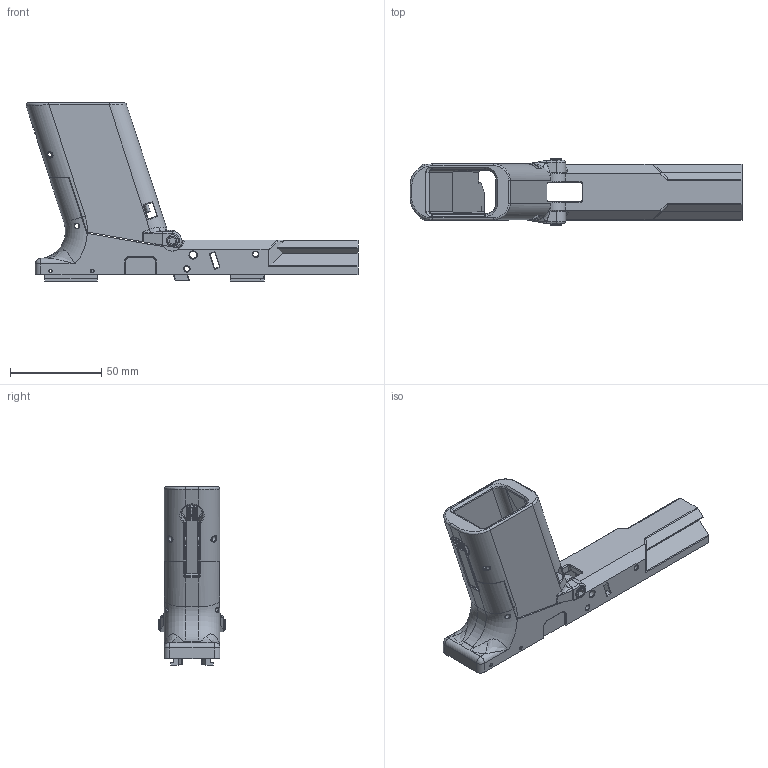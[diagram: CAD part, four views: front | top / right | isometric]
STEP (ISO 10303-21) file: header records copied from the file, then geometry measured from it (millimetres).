
FILE_DESCRIPTION(/* description */ (''),/* implementation_level */ '2;1');
FILE_NAME(/* name */ 'G19 FOLDING X FIXED.stp',/* time_stamp */ '2019-11-15T10:02:00+02:00',/* author */ (''),/* organization */ (''),/* preprocessor_version */ 'ST-DEVELOPER v15.2',/* originating_system */ 'Autodesk Translator Framework v2.0.0.5431',/* authorisation */ '');
FILE_SCHEMA (('AUTOMOTIVE_DESIGN { 1 0 10303 214 3 1 1 }'));
Length unit declared in the file: centimetre
Products named in the file (1): FOLDING X V5 FIXED
Bounding box: 181.62 x 36.6 x 97.38 mm (x, y, z)
Volume: 97898.8 mm3; surface area: 54978.3 mm2
Topology: 10 solids, 11 shells, 1273 faces, 3184 edges, 1898 vertices
Faces by surface type: cylinder 473, plane 355, bspline 222, torus 127, sphere 52, cone 44
Full cylindrical faces by diameter (mm): 1.655 x8, 1.8 x1, 2.557 x2, 3 x7, 3.057 x4, 3.06 x3, 4 x1, 4.011 x1, 4.042 x4, 6 x2, 6.5 x2
Entity records: 43507 total; most frequent: CARTESIAN_POINT 14144, ORIENTED_EDGE 6130, DIRECTION 6060, EDGE_CURVE 3065, AXIS2_PLACEMENT_3D 2329, VERTEX_POINT 1881, EDGE_LOOP 1418, LINE 1402
